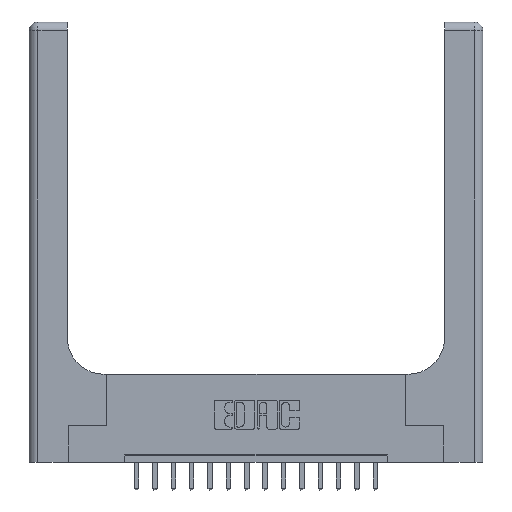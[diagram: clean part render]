
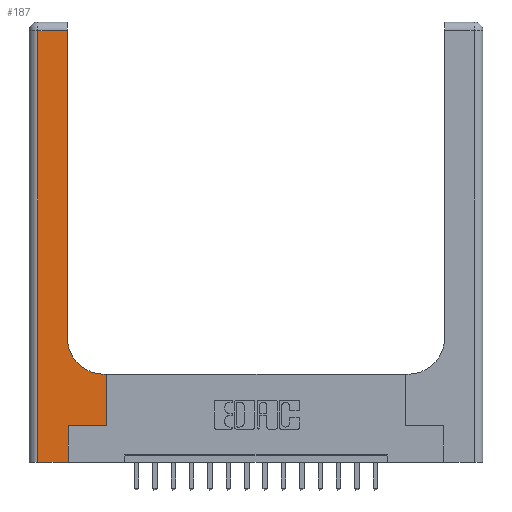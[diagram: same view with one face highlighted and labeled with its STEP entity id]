
A CAD part, top view. The second image highlights one B-rep face of the part: STEP entity #187.
In plain terms, the highlighted planar face has unit normal (0, 0, 1).
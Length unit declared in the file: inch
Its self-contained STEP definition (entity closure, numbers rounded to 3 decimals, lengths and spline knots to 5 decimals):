
#15 = VERTEX_POINT ( 'NONE', #15260 ) ;
#187 = ADVANCED_FACE ( 'NONE', ( #11634 ), #223, .F. ) ;
#223 = PLANE ( 'NONE',  #7931 ) ;
#517 = DIRECTION ( 'NONE',  ( 0., 0., -1. ) ) ;
#766 = VECTOR ( 'NONE', #1202, 39.37008 ) ;
#916 = VERTEX_POINT ( 'NONE', #14172 ) ;
#1188 = DIRECTION ( 'NONE',  ( 1., 0., 0. ) ) ;
#1202 = DIRECTION ( 'NONE',  ( -1., 0., 0. ) ) ;
#1655 = CARTESIAN_POINT ( 'NONE',  ( 0., 3., 0.37 ) ) ;
#1804 = LINE ( 'NONE', #10063, #2250 ) ;
#2090 = DIRECTION ( 'NONE',  ( -1., 0., 0. ) ) ;
#2250 = VECTOR ( 'NONE', #4737, 39.37008 ) ;
#2404 = EDGE_LOOP ( 'NONE', ( #7187, #12921, #3500, #15503, #7715, #7828, #17770, #12993, #16266 ) ) ;
#2501 = LINE ( 'NONE', #12207, #6998 ) ;
#2596 = EDGE_CURVE ( 'NONE', #10196, #4345, #15090, .T. ) ;
#2952 = CARTESIAN_POINT ( 'NONE',  ( 0.528, 0.25, 0.37 ) ) ;
#3209 = VECTOR ( 'NONE', #15759, 39.37008 ) ;
#3281 = CIRCLE ( 'NONE', #11364, 0.25 ) ;
#3500 = ORIENTED_EDGE ( 'NONE', *, *, #10085, .T. ) ;
#3980 = VECTOR ( 'NONE', #9740, 39.37008 ) ;
#4012 = LINE ( 'NONE', #12425, #4455 ) ;
#4072 = EDGE_CURVE ( 'NONE', #4345, #9535, #4677, .T. ) ;
#4250 = CARTESIAN_POINT ( 'NONE',  ( 0.26, 3., 0.37 ) ) ;
#4320 = EDGE_CURVE ( 'NONE', #15, #4377, #15181, .T. ) ;
#4345 = VERTEX_POINT ( 'NONE', #10775 ) ;
#4377 = VERTEX_POINT ( 'NONE', #5368 ) ;
#4427 = EDGE_CURVE ( 'NONE', #17128, #10196, #2501, .T. ) ;
#4455 = VECTOR ( 'NONE', #13940, 39.37008 ) ;
#4563 = EDGE_CURVE ( 'NONE', #5423, #15, #14519, .T. ) ;
#4677 = LINE ( 'NONE', #7472, #3209 ) ;
#4737 = DIRECTION ( 'NONE',  ( 0., 1., 0. ) ) ;
#4819 = CARTESIAN_POINT ( 'NONE',  ( 0.26, 0.85, 0.37 ) ) ;
#5368 = CARTESIAN_POINT ( 'NONE',  ( 0.06, 2.94, 0.37 ) ) ;
#5378 = VECTOR ( 'NONE', #11875, 39.37008 ) ;
#5423 = VERTEX_POINT ( 'NONE', #4819 ) ;
#5675 = CARTESIAN_POINT ( 'NONE',  ( 0.265, 0., 0.37 ) ) ;
#5727 = DIRECTION ( 'NONE',  ( 0., 1., 0. ) ) ;
#6298 = EDGE_CURVE ( 'NONE', #916, #5423, #3281, .T. ) ;
#6998 = VECTOR ( 'NONE', #16222, 39.37008 ) ;
#7153 = EDGE_CURVE ( 'NONE', #16477, #916, #12664, .T. ) ;
#7187 = ORIENTED_EDGE ( 'NONE', *, *, #4563, .T. ) ;
#7472 = CARTESIAN_POINT ( 'NONE',  ( 0.265, 0.25, 0.37 ) ) ;
#7497 = CARTESIAN_POINT ( 'NONE',  ( 0.265, 0., 0.37 ) ) ;
#7715 = ORIENTED_EDGE ( 'NONE', *, *, #2596, .T. ) ;
#7828 = ORIENTED_EDGE ( 'NONE', *, *, #4072, .T. ) ;
#7862 = CARTESIAN_POINT ( 'NONE',  ( 0.51, 0.85, 0.37 ) ) ;
#7931 = AXIS2_PLACEMENT_3D ( 'NONE', #1655, #517, #2090 ) ;
#8698 = CARTESIAN_POINT ( 'NONE',  ( 0.528, 0.6, 0.37 ) ) ;
#9282 = CARTESIAN_POINT ( 'NONE',  ( 0., 2.94, 0.37 ) ) ;
#9535 = VERTEX_POINT ( 'NONE', #2952 ) ;
#9740 = DIRECTION ( 'NONE',  ( 0., 1., 0. ) ) ;
#10063 = CARTESIAN_POINT ( 'NONE',  ( 0.528, 0.25, 0.37 ) ) ;
#10085 = EDGE_CURVE ( 'NONE', #4377, #17128, #4012, .T. ) ;
#10196 = VERTEX_POINT ( 'NONE', #7497 ) ;
#10775 = CARTESIAN_POINT ( 'NONE',  ( 0.265, 0.25, 0.37 ) ) ;
#11364 = AXIS2_PLACEMENT_3D ( 'NONE', #7862, #17511, #1188 ) ;
#11586 = EDGE_CURVE ( 'NONE', #9535, #16477, #1804, .T. ) ;
#11634 = FACE_OUTER_BOUND ( 'NONE', #2404, .T. ) ;
#11875 = DIRECTION ( 'NONE',  ( -1., 0., 0. ) ) ;
#12207 = CARTESIAN_POINT ( 'NONE',  ( 0., 0., 0.37 ) ) ;
#12425 = CARTESIAN_POINT ( 'NONE',  ( 0.06, 3., 0.37 ) ) ;
#12664 = LINE ( 'NONE', #13235, #5378 ) ;
#12921 = ORIENTED_EDGE ( 'NONE', *, *, #4320, .T. ) ;
#12993 = ORIENTED_EDGE ( 'NONE', *, *, #7153, .T. ) ;
#13235 = CARTESIAN_POINT ( 'NONE',  ( 0.26, 0.6, 0.37 ) ) ;
#13940 = DIRECTION ( 'NONE',  ( 0., -1., 0. ) ) ;
#14172 = CARTESIAN_POINT ( 'NONE',  ( 0.51, 0.6, 0.37 ) ) ;
#14519 = LINE ( 'NONE', #4250, #3980 ) ;
#14671 = VECTOR ( 'NONE', #5727, 39.37008 ) ;
#15090 = LINE ( 'NONE', #5675, #14671 ) ;
#15181 = LINE ( 'NONE', #9282, #766 ) ;
#15260 = CARTESIAN_POINT ( 'NONE',  ( 0.26, 2.94, 0.37 ) ) ;
#15503 = ORIENTED_EDGE ( 'NONE', *, *, #4427, .T. ) ;
#15638 = CARTESIAN_POINT ( 'NONE',  ( 0.06, 0., 0.37 ) ) ;
#15759 = DIRECTION ( 'NONE',  ( 1., 0., 0. ) ) ;
#16222 = DIRECTION ( 'NONE',  ( 1., 0., 0. ) ) ;
#16266 = ORIENTED_EDGE ( 'NONE', *, *, #6298, .T. ) ;
#16477 = VERTEX_POINT ( 'NONE', #8698 ) ;
#17128 = VERTEX_POINT ( 'NONE', #15638 ) ;
#17511 = DIRECTION ( 'NONE',  ( 0., 0., -1. ) ) ;
#17770 = ORIENTED_EDGE ( 'NONE', *, *, #11586, .T. ) ;
